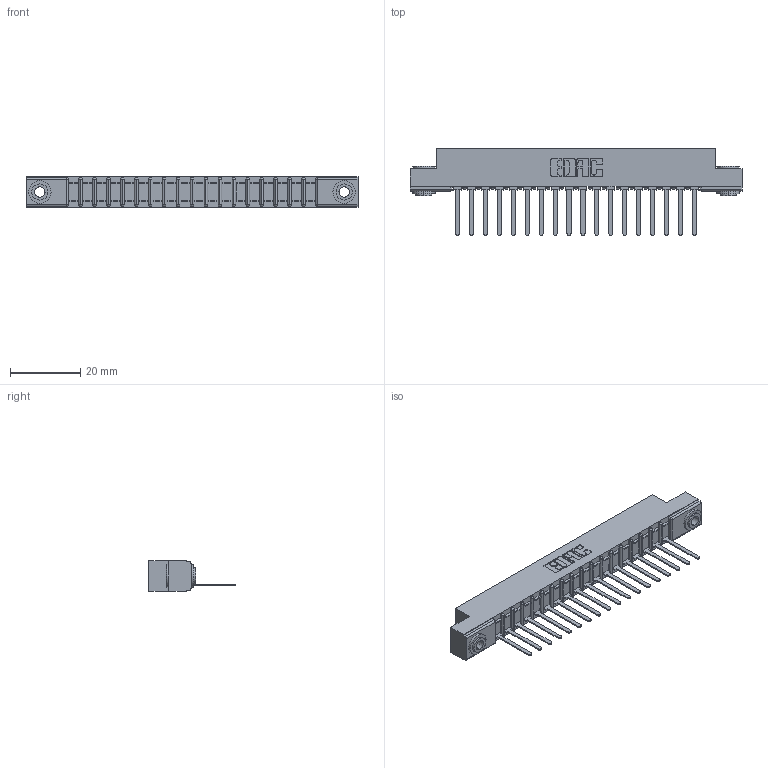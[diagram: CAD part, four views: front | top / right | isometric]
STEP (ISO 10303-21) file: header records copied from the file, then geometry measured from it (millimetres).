
FILE_DESCRIPTION (( 'STEP AP203' ), '1' );
FILE_NAME ('357-018-541-103.STEP', '2018-08-08T04:58:58', ( '' ), ( '' ), 'SwSTEP 2.0', 'SolidWorks 2016', '' );
FILE_SCHEMA (( 'CONFIG_CONTROL_DESIGN' ));
Length unit declared in the file: inch
Products named in the file (4): 307 Part_.156 Dia Mounting Holes; 307-290-002_541; 345-250-002_345-250-002-102; 357-018-541-103
Assembly tree (21 placements, depth 2):
  357-018-541-103
    307 Part_.156 Dia Mounting Holes
    307-290-002_541  x18
    345-250-002_345-250-002-102  x2
Bounding box: 94.34 x 24.59 x 8.71 mm (x, y, z)
Volume: 678.9 mm3; surface area: 11751.1 mm2
Topology: 20 solids, 21 shells, 1521 faces, 4611 edges, 3017 vertices
Faces by surface type: plane 904, cylinder 571, sphere 38, cone 8
Entity records: 20173 total; most frequent: CARTESIAN_POINT 3377, ORIENTED_EDGE 3358, DIRECTION 3307, EDGE_CURVE 1679, VECTOR 1267, LINE 1267, VERTEX_POINT 1090, AXIS2_PLACEMENT_3D 1020
